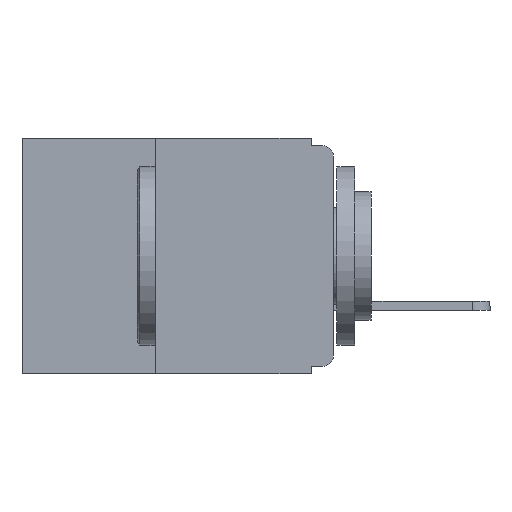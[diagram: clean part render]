
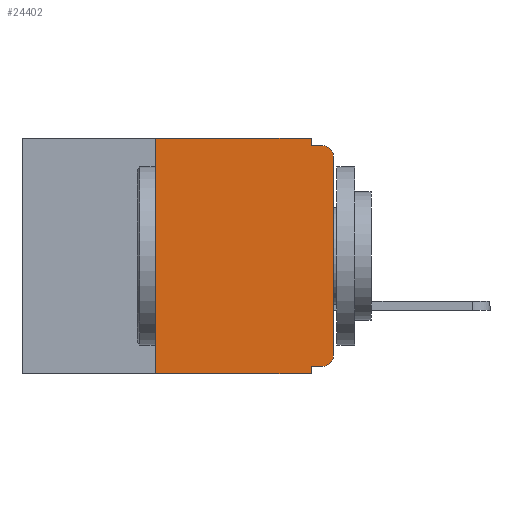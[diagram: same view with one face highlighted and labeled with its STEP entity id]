
A CAD part, left-side view. The second image highlights one B-rep face of the part: STEP entity #24402.
In plain terms, the highlighted planar face has unit normal (-1, 0, 0).
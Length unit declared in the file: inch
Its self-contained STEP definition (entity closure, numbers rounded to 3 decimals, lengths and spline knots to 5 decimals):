
#157 = AXIS2_PLACEMENT_3D ( 'NONE', #20981, #4872, #23692 ) ;
#1086 = EDGE_CURVE ( 'NONE', #19089, #19705, #15665, .T. ) ;
#1808 = DIRECTION ( 'NONE',  ( 1., 0., 0. ) ) ;
#1848 = ORIENTED_EDGE ( 'NONE', *, *, #14789, .F. ) ;
#3642 = EDGE_CURVE ( 'NONE', #30193, #7710, #25578, .T. ) ;
#3814 = LINE ( 'NONE', #8515, #31476 ) ;
#3870 = EDGE_CURVE ( 'NONE', #8321, #31951, #24321, .T. ) ;
#3952 = CARTESIAN_POINT ( 'NONE',  ( 0., 0.25, 0. ) ) ;
#4489 = PLANE ( 'NONE',  #22543 ) ;
#4872 = DIRECTION ( 'NONE',  ( -1., 0., 0. ) ) ;
#5045 = CARTESIAN_POINT ( 'NONE',  ( 0., 0.031, 0. ) ) ;
#5448 = VECTOR ( 'NONE', #34812, 39.37008 ) ;
#5897 = LINE ( 'NONE', #15223, #12227 ) ;
#6252 = VECTOR ( 'NONE', #13134, 39.37008 ) ;
#6703 = EDGE_CURVE ( 'NONE', #19089, #22507, #34689, .T. ) ;
#7144 = CARTESIAN_POINT ( 'NONE',  ( 0., 0.015, -0.025 ) ) ;
#7710 = VERTEX_POINT ( 'NONE', #13211 ) ;
#7722 = VECTOR ( 'NONE', #13905, 39.37008 ) ;
#7954 = EDGE_CURVE ( 'NONE', #26344, #30193, #29186, .T. ) ;
#8321 = VERTEX_POINT ( 'NONE', #18530 ) ;
#8515 = CARTESIAN_POINT ( 'NONE',  ( 0., 0., 0. ) ) ;
#8689 = ORIENTED_EDGE ( 'NONE', *, *, #14599, .F. ) ;
#8995 = DIRECTION ( 'NONE',  ( 0., 0., -1. ) ) ;
#9862 = DIRECTION ( 'NONE',  ( 0., 0., -1. ) ) ;
#10388 = ORIENTED_EDGE ( 'NONE', *, *, #1086, .F. ) ;
#10782 = CARTESIAN_POINT ( 'NONE',  ( 0., 0.437, 0. ) ) ;
#10937 = VECTOR ( 'NONE', #11441, 39.37008 ) ;
#11441 = DIRECTION ( 'NONE',  ( 0., 1., 0. ) ) ;
#11447 = CARTESIAN_POINT ( 'NONE',  ( 0., 0., -0.32 ) ) ;
#12227 = VECTOR ( 'NONE', #31220, 39.37008 ) ;
#12349 = EDGE_CURVE ( 'NONE', #32302, #7710, #16576, .T. ) ;
#12616 = LINE ( 'NONE', #10782, #5448 ) ;
#12730 = CARTESIAN_POINT ( 'NONE',  ( 0., 0.031, -0.33 ) ) ;
#12915 = CARTESIAN_POINT ( 'NONE',  ( 0., 0.437, -0.33 ) ) ;
#12937 = CIRCLE ( 'NONE', #157, 0.015 ) ;
#13134 = DIRECTION ( 'NONE',  ( 0., -1., 0. ) ) ;
#13211 = CARTESIAN_POINT ( 'NONE',  ( 0., 0.015, -0.01 ) ) ;
#13905 = DIRECTION ( 'NONE',  ( 0., 0., 1. ) ) ;
#14226 = CARTESIAN_POINT ( 'NONE',  ( 0., 0.25, -0.33 ) ) ;
#14599 = EDGE_CURVE ( 'NONE', #31951, #22507, #5897, .T. ) ;
#14789 = EDGE_CURVE ( 'NONE', #19705, #26344, #12616, .T. ) ;
#15223 = CARTESIAN_POINT ( 'NONE',  ( 0., 0.031, -0.33 ) ) ;
#15345 = CARTESIAN_POINT ( 'NONE',  ( 0., 0., -0.01 ) ) ;
#15376 = DIRECTION ( 'NONE',  ( 0., -1., 0. ) ) ;
#15665 = LINE ( 'NONE', #33375, #7722 ) ;
#15822 = EDGE_CURVE ( 'NONE', #8321, #16778, #12937, .T. ) ;
#16460 = ORIENTED_EDGE ( 'NONE', *, *, #3870, .F. ) ;
#16576 = CIRCLE ( 'NONE', #30548, 0.015 ) ;
#16778 = VERTEX_POINT ( 'NONE', #19514 ) ;
#18486 = ORIENTED_EDGE ( 'NONE', *, *, #3642, .F. ) ;
#18530 = CARTESIAN_POINT ( 'NONE',  ( 0., 0.015, -0.32 ) ) ;
#18620 = CARTESIAN_POINT ( 'NONE',  ( 0., 0., -0.025 ) ) ;
#19089 = VERTEX_POINT ( 'NONE', #14226 ) ;
#19514 = CARTESIAN_POINT ( 'NONE',  ( 0., 0., -0.305 ) ) ;
#19638 = CARTESIAN_POINT ( 'NONE',  ( 0., 0.031, 0. ) ) ;
#19705 = VERTEX_POINT ( 'NONE', #3952 ) ;
#19929 = FACE_OUTER_BOUND ( 'NONE', #26858, .T. ) ;
#20057 = ORIENTED_EDGE ( 'NONE', *, *, #12349, .T. ) ;
#20698 = DIRECTION ( 'NONE',  ( 0., 0., -1. ) ) ;
#20981 = CARTESIAN_POINT ( 'NONE',  ( 0., 0.015, -0.305 ) ) ;
#21275 = VECTOR ( 'NONE', #8995, 39.37008 ) ;
#22480 = ORIENTED_EDGE ( 'NONE', *, *, #33616, .T. ) ;
#22507 = VERTEX_POINT ( 'NONE', #12730 ) ;
#22543 = AXIS2_PLACEMENT_3D ( 'NONE', #31293, #1808, #20698 ) ;
#22821 = CARTESIAN_POINT ( 'NONE',  ( 0., 0.031, -0.01 ) ) ;
#23692 = DIRECTION ( 'NONE',  ( 0., 0., -1. ) ) ;
#24321 = LINE ( 'NONE', #11447, #10937 ) ;
#24366 = ORIENTED_EDGE ( 'NONE', *, *, #7954, .F. ) ;
#24402 = ADVANCED_FACE ( 'NONE', ( #19929 ), #4489, .F. ) ;
#25417 = ORIENTED_EDGE ( 'NONE', *, *, #6703, .T. ) ;
#25578 = LINE ( 'NONE', #15345, #26408 ) ;
#25854 = DIRECTION ( 'NONE',  ( -1., 0., 0. ) ) ;
#26344 = VERTEX_POINT ( 'NONE', #5045 ) ;
#26408 = VECTOR ( 'NONE', #15376, 39.37008 ) ;
#26858 = EDGE_LOOP ( 'NONE', ( #22480, #20057, #18486, #24366, #1848, #10388, #25417, #8689, #16460, #33700 ) ) ;
#27208 = DIRECTION ( 'NONE',  ( 0., 0., 1. ) ) ;
#27884 = CARTESIAN_POINT ( 'NONE',  ( 0., 0.031, -0.32 ) ) ;
#29186 = LINE ( 'NONE', #19638, #21275 ) ;
#30193 = VERTEX_POINT ( 'NONE', #22821 ) ;
#30548 = AXIS2_PLACEMENT_3D ( 'NONE', #7144, #25854, #9862 ) ;
#31220 = DIRECTION ( 'NONE',  ( 0., 0., -1. ) ) ;
#31293 = CARTESIAN_POINT ( 'NONE',  ( 0., 0.437, 0. ) ) ;
#31476 = VECTOR ( 'NONE', #27208, 39.37008 ) ;
#31951 = VERTEX_POINT ( 'NONE', #27884 ) ;
#32302 = VERTEX_POINT ( 'NONE', #18620 ) ;
#33375 = CARTESIAN_POINT ( 'NONE',  ( 0., 0.25, -0.33 ) ) ;
#33616 = EDGE_CURVE ( 'NONE', #16778, #32302, #3814, .T. ) ;
#33700 = ORIENTED_EDGE ( 'NONE', *, *, #15822, .T. ) ;
#34689 = LINE ( 'NONE', #12915, #6252 ) ;
#34812 = DIRECTION ( 'NONE',  ( 0., -1., 0. ) ) ;
